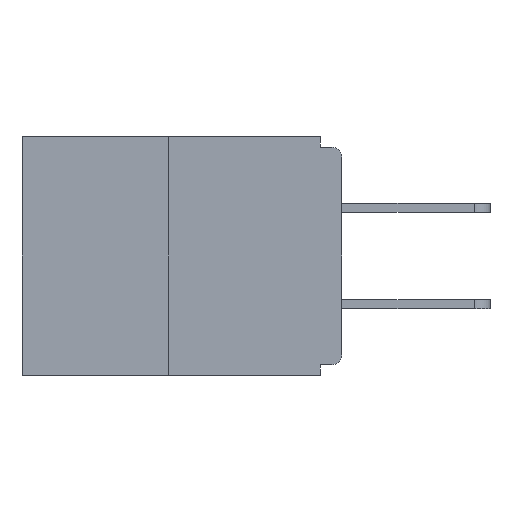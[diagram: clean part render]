
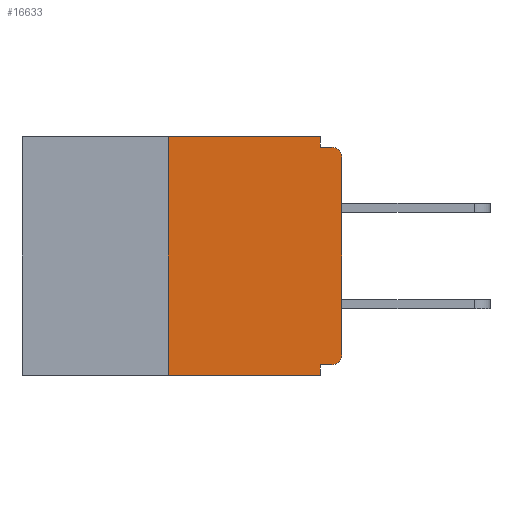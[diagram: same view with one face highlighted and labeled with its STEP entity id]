
A CAD part, left-side view. The second image highlights one B-rep face of the part: STEP entity #16633.
In plain terms, the highlighted planar face has unit normal (-1, 0, 0).
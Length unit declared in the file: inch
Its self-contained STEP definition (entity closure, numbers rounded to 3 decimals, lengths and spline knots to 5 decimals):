
#335 = LINE ( 'NONE', #3483, #10394 ) ;
#525 = VERTEX_POINT ( 'NONE', #2233 ) ;
#770 = VERTEX_POINT ( 'NONE', #3490 ) ;
#827 = ORIENTED_EDGE ( 'NONE', *, *, #13277, .T. ) ;
#908 = CARTESIAN_POINT ( 'NONE',  ( 0., 0.015, -0.03 ) ) ;
#924 = CARTESIAN_POINT ( 'NONE',  ( 0., 0., 0. ) ) ;
#1006 = CARTESIAN_POINT ( 'NONE',  ( 0., 0.46, 0. ) ) ;
#1071 = VERTEX_POINT ( 'NONE', #11457 ) ;
#1198 = CIRCLE ( 'NONE', #16298, 0.015 ) ;
#1608 = CARTESIAN_POINT ( 'NONE',  ( 0., 0.25, -0.343 ) ) ;
#1877 = CARTESIAN_POINT ( 'NONE',  ( 0., 0.031, 0. ) ) ;
#2051 = DIRECTION ( 'NONE',  ( 0., 0., -1. ) ) ;
#2140 = VECTOR ( 'NONE', #5563, 39.37008 ) ;
#2161 = ORIENTED_EDGE ( 'NONE', *, *, #8429, .F. ) ;
#2233 = CARTESIAN_POINT ( 'NONE',  ( 0., 0., -0.313 ) ) ;
#2364 = DIRECTION ( 'NONE',  ( 0., 0., 1. ) ) ;
#2400 = DIRECTION ( 'NONE',  ( -1., 0., 0. ) ) ;
#2418 = DIRECTION ( 'NONE',  ( 0., -1., 0. ) ) ;
#2878 = LINE ( 'NONE', #1877, #10568 ) ;
#2890 = VECTOR ( 'NONE', #7293, 39.37008 ) ;
#3195 = CIRCLE ( 'NONE', #6087, 0.015 ) ;
#3483 = CARTESIAN_POINT ( 'NONE',  ( 0., 0.031, -0.343 ) ) ;
#3490 = CARTESIAN_POINT ( 'NONE',  ( 0., 0.031, -0.015 ) ) ;
#3911 = VECTOR ( 'NONE', #17508, 39.37008 ) ;
#4127 = VERTEX_POINT ( 'NONE', #6274 ) ;
#4208 = DIRECTION ( 'NONE',  ( 0., -1., 0. ) ) ;
#4782 = EDGE_CURVE ( 'NONE', #770, #14960, #12028, .T. ) ;
#5060 = ORIENTED_EDGE ( 'NONE', *, *, #16606, .F. ) ;
#5253 = VERTEX_POINT ( 'NONE', #6677 ) ;
#5355 = ORIENTED_EDGE ( 'NONE', *, *, #6838, .T. ) ;
#5563 = DIRECTION ( 'NONE',  ( 0., 1., 0. ) ) ;
#6087 = AXIS2_PLACEMENT_3D ( 'NONE', #12142, #8087, #14996 ) ;
#6207 = ORIENTED_EDGE ( 'NONE', *, *, #12013, .F. ) ;
#6274 = CARTESIAN_POINT ( 'NONE',  ( 0., 0.25, 0. ) ) ;
#6547 = AXIS2_PLACEMENT_3D ( 'NONE', #12812, #14345, #10063 ) ;
#6562 = FACE_OUTER_BOUND ( 'NONE', #13909, .T. ) ;
#6677 = CARTESIAN_POINT ( 'NONE',  ( 0., 0.031, -0.343 ) ) ;
#6838 = EDGE_CURVE ( 'NONE', #17610, #525, #3195, .T. ) ;
#6952 = CARTESIAN_POINT ( 'NONE',  ( 0., 0., -0.328 ) ) ;
#7293 = DIRECTION ( 'NONE',  ( 0., 0., 1. ) ) ;
#7464 = CARTESIAN_POINT ( 'NONE',  ( 0., 0.031, 0. ) ) ;
#7506 = DIRECTION ( 'NONE',  ( 0., 0., -1. ) ) ;
#7741 = CARTESIAN_POINT ( 'NONE',  ( 0., 0.46, -0.343 ) ) ;
#7975 = VECTOR ( 'NONE', #4208, 39.37008 ) ;
#8086 = ORIENTED_EDGE ( 'NONE', *, *, #13153, .T. ) ;
#8087 = DIRECTION ( 'NONE',  ( -1., 0., 0. ) ) ;
#8429 = EDGE_CURVE ( 'NONE', #17610, #1071, #14314, .T. ) ;
#8979 = VERTEX_POINT ( 'NONE', #1608 ) ;
#9083 = ORIENTED_EDGE ( 'NONE', *, *, #4782, .F. ) ;
#9604 = CARTESIAN_POINT ( 'NONE',  ( 0., 0., -0.015 ) ) ;
#9778 = CARTESIAN_POINT ( 'NONE',  ( 0., 0.015, -0.328 ) ) ;
#10063 = DIRECTION ( 'NONE',  ( 0., 0., -1. ) ) ;
#10094 = VECTOR ( 'NONE', #2418, 39.37008 ) ;
#10394 = VECTOR ( 'NONE', #7506, 39.37008 ) ;
#10568 = VECTOR ( 'NONE', #2051, 39.37008 ) ;
#10589 = ORIENTED_EDGE ( 'NONE', *, *, #12926, .F. ) ;
#10642 = EDGE_CURVE ( 'NONE', #12873, #14960, #1198, .T. ) ;
#10776 = LINE ( 'NONE', #15525, #2890 ) ;
#11041 = EDGE_CURVE ( 'NONE', #8979, #4127, #10776, .T. ) ;
#11338 = ORIENTED_EDGE ( 'NONE', *, *, #10642, .T. ) ;
#11457 = CARTESIAN_POINT ( 'NONE',  ( 0., 0.031, -0.328 ) ) ;
#11519 = VERTEX_POINT ( 'NONE', #7464 ) ;
#11599 = LINE ( 'NONE', #924, #12454 ) ;
#12013 = EDGE_CURVE ( 'NONE', #11519, #770, #2878, .T. ) ;
#12028 = LINE ( 'NONE', #9604, #7975 ) ;
#12142 = CARTESIAN_POINT ( 'NONE',  ( 0., 0.015, -0.313 ) ) ;
#12454 = VECTOR ( 'NONE', #2364, 39.37008 ) ;
#12812 = CARTESIAN_POINT ( 'NONE',  ( 0., 0.46, 0. ) ) ;
#12868 = PLANE ( 'NONE',  #6547 ) ;
#12873 = VERTEX_POINT ( 'NONE', #16783 ) ;
#12926 = EDGE_CURVE ( 'NONE', #4127, #11519, #16721, .T. ) ;
#13153 = EDGE_CURVE ( 'NONE', #525, #12873, #11599, .T. ) ;
#13277 = EDGE_CURVE ( 'NONE', #8979, #5253, #13731, .T. ) ;
#13731 = LINE ( 'NONE', #7741, #10094 ) ;
#13909 = EDGE_LOOP ( 'NONE', ( #10589, #16238, #827, #5060, #2161, #5355, #8086, #11338, #9083, #6207 ) ) ;
#14314 = LINE ( 'NONE', #6952, #2140 ) ;
#14345 = DIRECTION ( 'NONE',  ( 1., 0., 0. ) ) ;
#14960 = VERTEX_POINT ( 'NONE', #16845 ) ;
#14996 = DIRECTION ( 'NONE',  ( 0., 0., -1. ) ) ;
#15525 = CARTESIAN_POINT ( 'NONE',  ( 0., 0.25, 0. ) ) ;
#16059 = DIRECTION ( 'NONE',  ( 0., 0., -1. ) ) ;
#16238 = ORIENTED_EDGE ( 'NONE', *, *, #11041, .F. ) ;
#16298 = AXIS2_PLACEMENT_3D ( 'NONE', #908, #2400, #16059 ) ;
#16606 = EDGE_CURVE ( 'NONE', #1071, #5253, #335, .T. ) ;
#16633 = ADVANCED_FACE ( 'NONE', ( #6562 ), #12868, .F. ) ;
#16721 = LINE ( 'NONE', #1006, #3911 ) ;
#16783 = CARTESIAN_POINT ( 'NONE',  ( 0., 0., -0.03 ) ) ;
#16845 = CARTESIAN_POINT ( 'NONE',  ( 0., 0.015, -0.015 ) ) ;
#17508 = DIRECTION ( 'NONE',  ( 0., -1., 0. ) ) ;
#17610 = VERTEX_POINT ( 'NONE', #9778 ) ;
